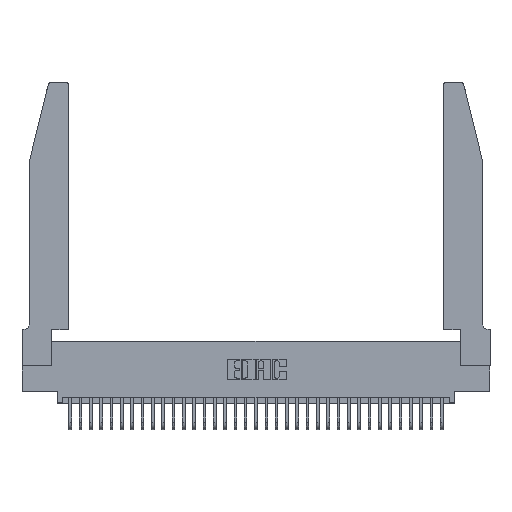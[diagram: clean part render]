
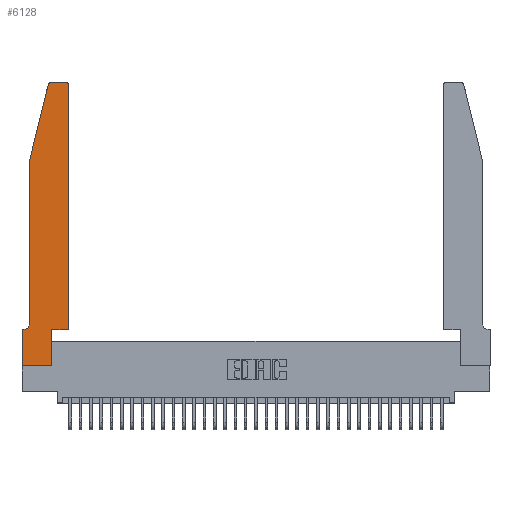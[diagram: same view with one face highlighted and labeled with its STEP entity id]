
A CAD part, top view. The second image highlights one B-rep face of the part: STEP entity #6128.
In plain terms, the highlighted planar face has unit normal (0, 0, 1).
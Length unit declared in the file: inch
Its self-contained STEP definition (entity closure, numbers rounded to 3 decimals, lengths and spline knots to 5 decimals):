
#331 = VECTOR ( 'NONE', #20930, 39.37008 ) ;
#1439 = EDGE_LOOP ( 'NONE', ( #11376, #32144, #31136, #17817, #3181, #31217, #11654, #11380, #22166, #24380, #30203, #14872 ) ) ;
#1528 = CARTESIAN_POINT ( 'NONE',  ( 0.0055, 0.42, 0.37 ) ) ;
#1567 = DIRECTION ( 'NONE',  ( -1., 0., 0. ) ) ;
#1920 = LINE ( 'NONE', #33068, #20917 ) ;
#2138 = EDGE_CURVE ( 'NONE', #15218, #22709, #24659, .T. ) ;
#2915 = EDGE_CURVE ( 'NONE', #12786, #18246, #8839, .T. ) ;
#3146 = LINE ( 'NONE', #19668, #29020 ) ;
#3181 = ORIENTED_EDGE ( 'NONE', *, *, #24290, .T. ) ;
#3562 = CARTESIAN_POINT ( 'NONE',  ( 0.0755, 2., 0.37 ) ) ;
#4107 = DIRECTION ( 'NONE',  ( -1., 0., 0. ) ) ;
#4272 = CARTESIAN_POINT ( 'NONE',  ( 0.4205, 2.75, 0.37 ) ) ;
#4653 = VERTEX_POINT ( 'NONE', #23117 ) ;
#5504 = VERTEX_POINT ( 'NONE', #15948 ) ;
#6128 = ADVANCED_FACE ( 'NONE', ( #25282 ), #9961, .T. ) ;
#6379 = CARTESIAN_POINT ( 'NONE',  ( 0.25487, 2.72718, 0.37 ) ) ;
#6995 = CARTESIAN_POINT ( 'NONE',  ( 0.284, 2.72, 0.37 ) ) ;
#7251 = LINE ( 'NONE', #15820, #331 ) ;
#7899 = CARTESIAN_POINT ( 'NONE',  ( 0.4205, 2.72, 0.37 ) ) ;
#8028 = VECTOR ( 'NONE', #13288, 39.37008 ) ;
#8091 = CARTESIAN_POINT ( 'NONE',  ( 0.2865, 0.35, 0.37 ) ) ;
#8839 = LINE ( 'NONE', #8091, #8028 ) ;
#9596 = DIRECTION ( 'NONE',  ( 1., 0., 0. ) ) ;
#9961 = PLANE ( 'NONE',  #18214 ) ;
#10059 = EDGE_CURVE ( 'NONE', #25433, #15218, #14961, .T. ) ;
#10077 = DIRECTION ( 'NONE',  ( 0., 0., 1. ) ) ;
#10116 = AXIS2_PLACEMENT_3D ( 'NONE', #7899, #25966, #10491 ) ;
#10491 = DIRECTION ( 'NONE',  ( 1., 0., 0. ) ) ;
#10905 = VECTOR ( 'NONE', #31238, 39.37008 ) ;
#11376 = ORIENTED_EDGE ( 'NONE', *, *, #26094, .T. ) ;
#11379 = EDGE_CURVE ( 'NONE', #18246, #13532, #1920, .T. ) ;
#11380 = ORIENTED_EDGE ( 'NONE', *, *, #25106, .T. ) ;
#11654 = ORIENTED_EDGE ( 'NONE', *, *, #20165, .T. ) ;
#12786 = VERTEX_POINT ( 'NONE', #14444 ) ;
#12892 = AXIS2_PLACEMENT_3D ( 'NONE', #6995, #25076, #9596 ) ;
#13288 = DIRECTION ( 'NONE',  ( 0., 1., 0. ) ) ;
#13316 = CARTESIAN_POINT ( 'NONE',  ( 0., 0., 0.37 ) ) ;
#13532 = VERTEX_POINT ( 'NONE', #32849 ) ;
#14444 = CARTESIAN_POINT ( 'NONE',  ( 0.2865, 0., 0.37 ) ) ;
#14664 = CARTESIAN_POINT ( 'NONE',  ( 0.4505, 0.35, 0.37 ) ) ;
#14872 = ORIENTED_EDGE ( 'NONE', *, *, #19810, .T. ) ;
#14961 = CIRCLE ( 'NONE', #12892, 0.03 ) ;
#15052 = DIRECTION ( 'NONE',  ( 1., 0., 0. ) ) ;
#15218 = VERTEX_POINT ( 'NONE', #6379 ) ;
#15292 = VECTOR ( 'NONE', #25043, 39.37008 ) ;
#15682 = CARTESIAN_POINT ( 'NONE',  ( 0.0755, 2., 0.37 ) ) ;
#15820 = CARTESIAN_POINT ( 'NONE',  ( 0., 0., 0.37 ) ) ;
#15894 = DIRECTION ( 'NONE',  ( 0., -1., 0. ) ) ;
#15948 = CARTESIAN_POINT ( 'NONE',  ( 0.0055, 0.35, 0.37 ) ) ;
#16081 = CARTESIAN_POINT ( 'NONE',  ( 0.2605, 2.75, 0.37 ) ) ;
#16085 = CARTESIAN_POINT ( 'NONE',  ( 0.0755, 2., 0.37 ) ) ;
#16346 = CARTESIAN_POINT ( 'NONE',  ( 0.2865, 0.35, 0.37 ) ) ;
#16659 = CARTESIAN_POINT ( 'NONE',  ( 0., 0., 0.37 ) ) ;
#16867 = LINE ( 'NONE', #3562, #30603 ) ;
#17323 = AXIS2_PLACEMENT_3D ( 'NONE', #1528, #19628, #4107 ) ;
#17817 = ORIENTED_EDGE ( 'NONE', *, *, #20060, .T. ) ;
#18095 = CIRCLE ( 'NONE', #10116, 0.03 ) ;
#18214 = AXIS2_PLACEMENT_3D ( 'NONE', #33189, #10077, #28145 ) ;
#18246 = VERTEX_POINT ( 'NONE', #16346 ) ;
#18607 = CARTESIAN_POINT ( 'NONE',  ( 0.4505, 2.72, 0.37 ) ) ;
#19619 = EDGE_CURVE ( 'NONE', #5504, #32303, #3146, .T. ) ;
#19628 = DIRECTION ( 'NONE',  ( 0., 0., -1. ) ) ;
#19668 = CARTESIAN_POINT ( 'NONE',  ( 0.0755, 0.35, 0.37 ) ) ;
#19715 = VECTOR ( 'NONE', #15894, 39.37008 ) ;
#19810 = EDGE_CURVE ( 'NONE', #22073, #28419, #18095, .T. ) ;
#20060 = EDGE_CURVE ( 'NONE', #22709, #4653, #16867, .T. ) ;
#20165 = EDGE_CURVE ( 'NONE', #32303, #29796, #33393, .T. ) ;
#20917 = VECTOR ( 'NONE', #15052, 39.37008 ) ;
#20930 = DIRECTION ( 'NONE',  ( 1., 0., 0. ) ) ;
#20960 = CARTESIAN_POINT ( 'NONE',  ( 0., 0.35, 0.37 ) ) ;
#21684 = DIRECTION ( 'NONE',  ( 0., -1., 0. ) ) ;
#22073 = VERTEX_POINT ( 'NONE', #18607 ) ;
#22166 = ORIENTED_EDGE ( 'NONE', *, *, #2915, .T. ) ;
#22709 = VERTEX_POINT ( 'NONE', #16085 ) ;
#22975 = LINE ( 'NONE', #14664, #15292 ) ;
#23117 = CARTESIAN_POINT ( 'NONE',  ( 0.0755, 0.42, 0.37 ) ) ;
#23752 = VECTOR ( 'NONE', #31612, 39.37008 ) ;
#24290 = EDGE_CURVE ( 'NONE', #4653, #5504, #24712, .T. ) ;
#24380 = ORIENTED_EDGE ( 'NONE', *, *, #11379, .T. ) ;
#24659 = LINE ( 'NONE', #15682, #10905 ) ;
#24712 = CIRCLE ( 'NONE', #17323, 0.07 ) ;
#25043 = DIRECTION ( 'NONE',  ( 0., 1., 0. ) ) ;
#25076 = DIRECTION ( 'NONE',  ( 0., 0., 1. ) ) ;
#25106 = EDGE_CURVE ( 'NONE', #29796, #12786, #7251, .T. ) ;
#25190 = CARTESIAN_POINT ( 'NONE',  ( 0.284, 2.75, 0.37 ) ) ;
#25282 = FACE_OUTER_BOUND ( 'NONE', #1439, .T. ) ;
#25433 = VERTEX_POINT ( 'NONE', #25190 ) ;
#25769 = EDGE_CURVE ( 'NONE', #13532, #22073, #22975, .T. ) ;
#25966 = DIRECTION ( 'NONE',  ( 0., 0., 1. ) ) ;
#26094 = EDGE_CURVE ( 'NONE', #28419, #25433, #30599, .T. ) ;
#28145 = DIRECTION ( 'NONE',  ( 1., 0., 0. ) ) ;
#28419 = VERTEX_POINT ( 'NONE', #4272 ) ;
#29020 = VECTOR ( 'NONE', #1567, 39.37008 ) ;
#29796 = VERTEX_POINT ( 'NONE', #16659 ) ;
#30203 = ORIENTED_EDGE ( 'NONE', *, *, #25769, .T. ) ;
#30599 = LINE ( 'NONE', #16081, #23752 ) ;
#30603 = VECTOR ( 'NONE', #21684, 39.37008 ) ;
#31136 = ORIENTED_EDGE ( 'NONE', *, *, #2138, .T. ) ;
#31217 = ORIENTED_EDGE ( 'NONE', *, *, #19619, .T. ) ;
#31238 = DIRECTION ( 'NONE',  ( -0.239, -0.971, 0. ) ) ;
#31612 = DIRECTION ( 'NONE',  ( -1., 0., 0. ) ) ;
#32144 = ORIENTED_EDGE ( 'NONE', *, *, #10059, .T. ) ;
#32303 = VERTEX_POINT ( 'NONE', #20960 ) ;
#32849 = CARTESIAN_POINT ( 'NONE',  ( 0.4505, 0.35, 0.37 ) ) ;
#33068 = CARTESIAN_POINT ( 'NONE',  ( 0.4505, 0.35, 0.37 ) ) ;
#33189 = CARTESIAN_POINT ( 'NONE',  ( 0., 0.35, 0.37 ) ) ;
#33393 = LINE ( 'NONE', #13316, #19715 ) ;
